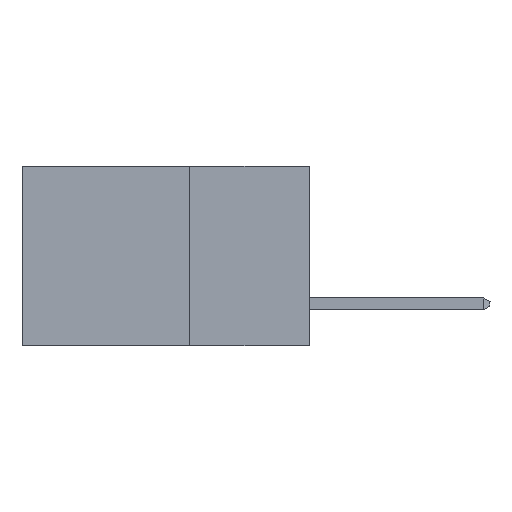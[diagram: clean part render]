
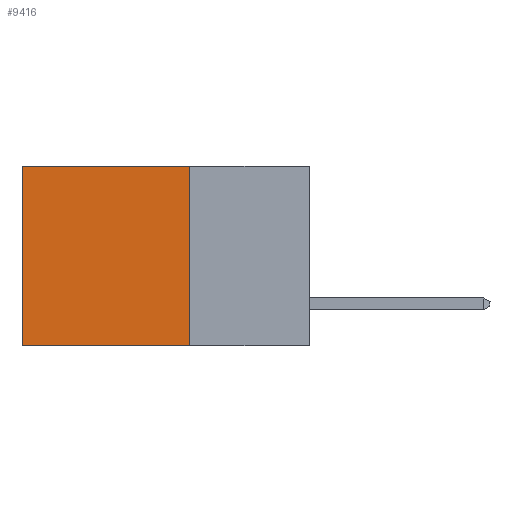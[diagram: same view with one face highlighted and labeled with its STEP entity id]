
A CAD part, left-side view. The second image highlights one B-rep face of the part: STEP entity #9416.
In plain terms, the highlighted planar face has unit normal (-1, 0, 0).
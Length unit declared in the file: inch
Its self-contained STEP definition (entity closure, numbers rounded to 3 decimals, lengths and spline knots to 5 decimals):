
#454 = DIRECTION ( 'NONE',  ( 0., 1., 0. ) ) ;
#1120 = LINE ( 'NONE', #11078, #8794 ) ;
#1175 = CARTESIAN_POINT ( 'NONE',  ( 0.2875, 0.25, 0. ) ) ;
#1951 = VECTOR ( 'NONE', #3511, 39.37008 ) ;
#2364 = CARTESIAN_POINT ( 'NONE',  ( 0.2875, 0.25, -0.375 ) ) ;
#2730 = CARTESIAN_POINT ( 'NONE',  ( 0.2875, 0.25, -0.375 ) ) ;
#3174 = ORIENTED_EDGE ( 'NONE', *, *, #14571, .T. ) ;
#3208 = DIRECTION ( 'NONE',  ( 1., 0., 0. ) ) ;
#3511 = DIRECTION ( 'NONE',  ( 0., 0., -1. ) ) ;
#3762 = LINE ( 'NONE', #2364, #1951 ) ;
#4130 = LINE ( 'NONE', #12246, #12897 ) ;
#4182 = VERTEX_POINT ( 'NONE', #11804 ) ;
#4216 = AXIS2_PLACEMENT_3D ( 'NONE', #10236, #3208, #5623 ) ;
#4499 = EDGE_CURVE ( 'NONE', #4182, #4719, #11690, .T. ) ;
#4719 = VERTEX_POINT ( 'NONE', #14202 ) ;
#4910 = VERTEX_POINT ( 'NONE', #12352 ) ;
#5114 = VERTEX_POINT ( 'NONE', #1175 ) ;
#5469 = VECTOR ( 'NONE', #454, 39.37008 ) ;
#5623 = DIRECTION ( 'NONE',  ( 0., 0., -1. ) ) ;
#6313 = EDGE_CURVE ( 'NONE', #5114, #4182, #3762, .T. ) ;
#6535 = EDGE_LOOP ( 'NONE', ( #11074, #14979, #14729, #3174 ) ) ;
#6691 = PLANE ( 'NONE',  #4216 ) ;
#8794 = VECTOR ( 'NONE', #14613, 39.37008 ) ;
#9287 = EDGE_CURVE ( 'NONE', #4910, #4719, #1120, .T. ) ;
#9416 = ADVANCED_FACE ( 'NONE', ( #14443 ), #6691, .F. ) ;
#9959 = DIRECTION ( 'NONE',  ( 0., 1., 0. ) ) ;
#10236 = CARTESIAN_POINT ( 'NONE',  ( 0.2875, 0.25, -0.375 ) ) ;
#11074 = ORIENTED_EDGE ( 'NONE', *, *, #9287, .T. ) ;
#11078 = CARTESIAN_POINT ( 'NONE',  ( 0.2875, 0.6, -0.375 ) ) ;
#11690 = LINE ( 'NONE', #2730, #5469 ) ;
#11804 = CARTESIAN_POINT ( 'NONE',  ( 0.2875, 0.25, -0.375 ) ) ;
#12246 = CARTESIAN_POINT ( 'NONE',  ( 0.2875, 0.25, 0. ) ) ;
#12352 = CARTESIAN_POINT ( 'NONE',  ( 0.2875, 0.6, 0. ) ) ;
#12897 = VECTOR ( 'NONE', #9959, 39.37008 ) ;
#14202 = CARTESIAN_POINT ( 'NONE',  ( 0.2875, 0.6, -0.375 ) ) ;
#14443 = FACE_OUTER_BOUND ( 'NONE', #6535, .T. ) ;
#14571 = EDGE_CURVE ( 'NONE', #5114, #4910, #4130, .T. ) ;
#14613 = DIRECTION ( 'NONE',  ( 0., 0., -1. ) ) ;
#14729 = ORIENTED_EDGE ( 'NONE', *, *, #6313, .F. ) ;
#14979 = ORIENTED_EDGE ( 'NONE', *, *, #4499, .F. ) ;
